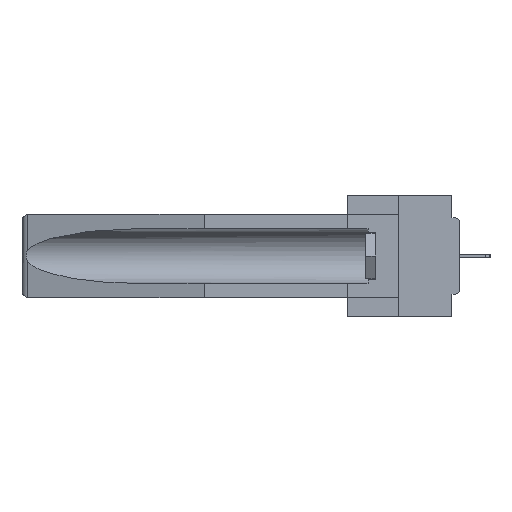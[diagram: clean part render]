
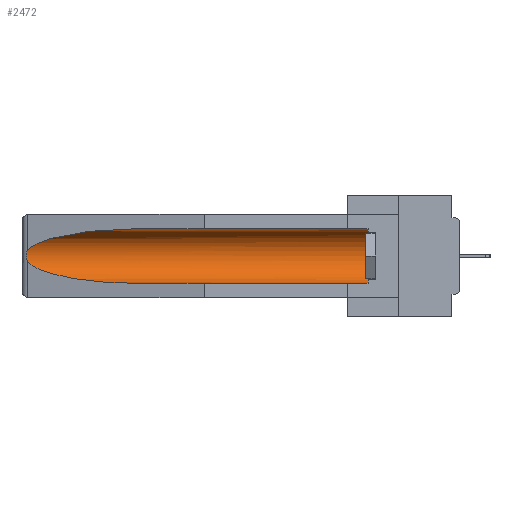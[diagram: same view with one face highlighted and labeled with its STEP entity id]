
A CAD part, left-side view. The second image highlights one B-rep face of the part: STEP entity #2472.
In plain terms, the highlighted cylindrical face has radius 2.857 mm (diameter 5.715 mm), a partial arc.
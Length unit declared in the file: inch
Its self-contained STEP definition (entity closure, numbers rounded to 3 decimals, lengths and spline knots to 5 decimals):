
#181 = EDGE_CURVE ( 'NONE', #25980, #3811, #8654, .T. ) ;
#331 = CARTESIAN_POINT ( 'NONE',  ( 0.26537, 1.52718, -0.14972 ) ) ;
#527 = VECTOR ( 'NONE', #7352, 39.37008 ) ;
#1169 = ORIENTED_EDGE ( 'NONE', *, *, #31866, .T. ) ;
#1755 = DIRECTION ( 'NONE',  ( 0., 1., 0. ) ) ;
#1841 = CARTESIAN_POINT ( 'NONE',  ( 0.155, -0.30754, -0.284 ) ) ;
#2472 = ADVANCED_FACE ( 'NONE', ( #38573 ), #35554, .F. ) ;
#2637 = VERTEX_POINT ( 'NONE', #19140 ) ;
#3710 = CARTESIAN_POINT ( 'NONE',  ( 0.21114, 1.30732, -0.059 ) ) ;
#3811 = VERTEX_POINT ( 'NONE', #3980 ) ;
#3980 = CARTESIAN_POINT ( 'NONE',  ( 0.155, 1.07973, -0.284 ) ) ;
#5391 = CARTESIAN_POINT ( 'NONE',  ( 0.2673, 1.5327, -0.16383 ) ) ;
#5588 = CARTESIAN_POINT ( 'NONE',  ( 0.2675, 1.53308, -0.16763 ) ) ;
#6048 =( BOUNDED_CURVE ( )  B_SPLINE_CURVE ( 3, ( #34646, #3710, #10211, #25382 ),
 .UNSPECIFIED., .F., .F. ) 
 B_SPLINE_CURVE_WITH_KNOTS ( ( 4, 4 ),
 ( 4.71239, 6.08839 ),
 .UNSPECIFIED. ) 
 CURVE ( )  GEOMETRIC_REPRESENTATION_ITEM ( )  RATIONAL_B_SPLINE_CURVE ( ( 1., 0.848, 0.848, 1. ) ) 
 REPRESENTATION_ITEM ( '' )  );
#6558 = ORIENTED_EDGE ( 'NONE', *, *, #33483, .T. ) ;
#7045 = DIRECTION ( 'NONE',  ( 0., -1., 0. ) ) ;
#7352 = DIRECTION ( 'NONE',  ( 0., 1., 0. ) ) ;
#7710 = ORIENTED_EDGE ( 'NONE', *, *, #13704, .F. ) ;
#7885 = ORIENTED_EDGE ( 'NONE', *, *, #35452, .T. ) ;
#8654 =( BOUNDED_CURVE ( )  B_SPLINE_CURVE ( 3, ( #29255, #29067, #19751, #31883 ),
 .UNSPECIFIED., .F., .F. ) 
 B_SPLINE_CURVE_WITH_KNOTS ( ( 4, 4 ),
 ( 0.1948, 1.5708 ),
 .UNSPECIFIED. ) 
 CURVE ( )  GEOMETRIC_REPRESENTATION_ITEM ( )  RATIONAL_B_SPLINE_CURVE ( ( 1., 0.848, 0.848, 1. ) ) 
 REPRESENTATION_ITEM ( '' )  );
#9030 = CARTESIAN_POINT ( 'NONE',  ( 0.26537, 1.52718, -0.19328 ) ) ;
#9231 = VERTEX_POINT ( 'NONE', #11738 ) ;
#10211 = CARTESIAN_POINT ( 'NONE',  ( 0.25451, 1.48313, -0.09465 ) ) ;
#10993 = LINE ( 'NONE', #1841, #527 ) ;
#11209 = CIRCLE ( 'NONE', #14394, 0.1125 ) ;
#11738 = CARTESIAN_POINT ( 'NONE',  ( 0.155, 0.126, -0.059 ) ) ;
#12406 = EDGE_CURVE ( 'NONE', #9231, #2637, #32929, .T. ) ;
#13704 = EDGE_CURVE ( 'NONE', #16785, #3811, #10993, .T. ) ;
#14394 = AXIS2_PLACEMENT_3D ( 'NONE', #19161, #7045, #19381 ) ;
#14500 = CARTESIAN_POINT ( 'NONE',  ( 0.155, -0.30754, -0.059 ) ) ;
#14871 = CARTESIAN_POINT ( 'NONE',  ( 0.26655, 1.53094, -0.18657 ) ) ;
#16785 = VERTEX_POINT ( 'NONE', #23015 ) ;
#18124 = CARTESIAN_POINT ( 'NONE',  ( 0.26597, 1.52961, -0.15275 ) ) ;
#19140 = CARTESIAN_POINT ( 'NONE',  ( 0.155, 1.07973, -0.059 ) ) ;
#19161 = CARTESIAN_POINT ( 'NONE',  ( 0.155, 0.126, -0.1715 ) ) ;
#19381 = DIRECTION ( 'NONE',  ( 0., 0., 1. ) ) ;
#19407 = ORIENTED_EDGE ( 'NONE', *, *, #181, .T. ) ;
#19751 = CARTESIAN_POINT ( 'NONE',  ( 0.21114, 1.30732, -0.284 ) ) ;
#21148 = CARTESIAN_POINT ( 'NONE',  ( 0.26537, 1.52718, -0.14972 ) ) ;
#23015 = CARTESIAN_POINT ( 'NONE',  ( 0.155, 0.126, -0.284 ) ) ;
#23480 = B_SPLINE_CURVE_WITH_KNOTS ( 'NONE', 3,
 ( #21148, #18124, #35913, #5391, #5588, #39735, #27411, #14871, #39552, #9030 ),
 .UNSPECIFIED., .F., .F.,
 ( 4, 2, 2, 2, 4 ),
 ( 0., 0.00029, 0.00058, 0.00087, 0.00117 ),
 .UNSPECIFIED. ) ;
#24226 = ORIENTED_EDGE ( 'NONE', *, *, #12406, .T. ) ;
#25382 = CARTESIAN_POINT ( 'NONE',  ( 0.26537, 1.52718, -0.14972 ) ) ;
#25980 = VERTEX_POINT ( 'NONE', #38842 ) ;
#26050 = EDGE_LOOP ( 'NONE', ( #7885, #6558, #19407, #7710, #1169, #24226 ) ) ;
#26870 = DIRECTION ( 'NONE',  ( 0., 1., 0. ) ) ;
#27411 = CARTESIAN_POINT ( 'NONE',  ( 0.2673, 1.53269, -0.17917 ) ) ;
#29067 = CARTESIAN_POINT ( 'NONE',  ( 0.25451, 1.48313, -0.24835 ) ) ;
#29255 = CARTESIAN_POINT ( 'NONE',  ( 0.26537, 1.52718, -0.19328 ) ) ;
#29472 = CARTESIAN_POINT ( 'NONE',  ( 0.155, -0.30754, -0.1715 ) ) ;
#31866 = EDGE_CURVE ( 'NONE', #16785, #9231, #11209, .T. ) ;
#31883 = CARTESIAN_POINT ( 'NONE',  ( 0.155, 1.07973, -0.284 ) ) ;
#32929 = LINE ( 'NONE', #14500, #35596 ) ;
#33483 = EDGE_CURVE ( 'NONE', #36317, #25980, #23480, .T. ) ;
#34646 = CARTESIAN_POINT ( 'NONE',  ( 0.155, 1.07973, -0.059 ) ) ;
#35452 = EDGE_CURVE ( 'NONE', #2637, #36317, #6048, .T. ) ;
#35554 = CYLINDRICAL_SURFACE ( 'NONE', #39601, 0.1125 ) ;
#35596 = VECTOR ( 'NONE', #26870, 39.37008 ) ;
#35739 = DIRECTION ( 'NONE',  ( 0., 0., 1. ) ) ;
#35913 = CARTESIAN_POINT ( 'NONE',  ( 0.26654, 1.53092, -0.15636 ) ) ;
#36317 = VERTEX_POINT ( 'NONE', #331 ) ;
#38573 = FACE_OUTER_BOUND ( 'NONE', #26050, .T. ) ;
#38842 = CARTESIAN_POINT ( 'NONE',  ( 0.26537, 1.52718, -0.19328 ) ) ;
#39552 = CARTESIAN_POINT ( 'NONE',  ( 0.26597, 1.5296, -0.19026 ) ) ;
#39601 = AXIS2_PLACEMENT_3D ( 'NONE', #29472, #1755, #35739 ) ;
#39735 = CARTESIAN_POINT ( 'NONE',  ( 0.2675, 1.53308, -0.17534 ) ) ;
